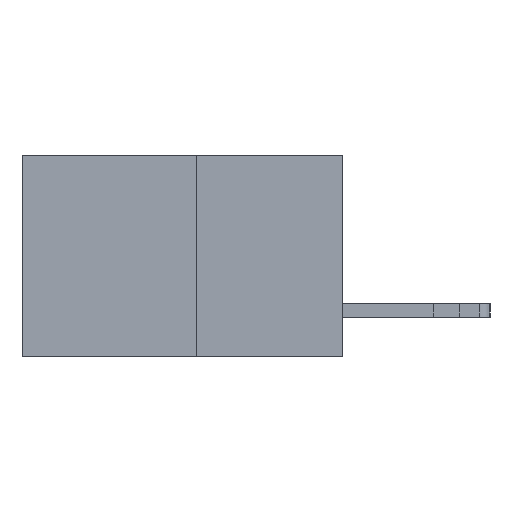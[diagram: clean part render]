
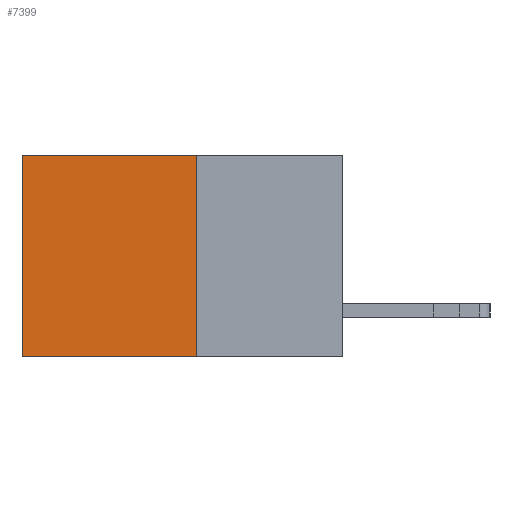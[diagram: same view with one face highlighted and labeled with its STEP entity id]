
A CAD part, left-side view. The second image highlights one B-rep face of the part: STEP entity #7399.
In plain terms, the highlighted planar face has unit normal (-1, 0, 0).
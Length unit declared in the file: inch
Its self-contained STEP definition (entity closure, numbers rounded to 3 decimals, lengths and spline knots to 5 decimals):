
#207 = VECTOR ( 'NONE', #7858, 39.37008 ) ;
#418 = CARTESIAN_POINT ( 'NONE',  ( 0.277, 0.59, 0. ) ) ;
#1033 = VECTOR ( 'NONE', #6911, 39.37008 ) ;
#1538 = CARTESIAN_POINT ( 'NONE',  ( 0.277, 0.59, -0.37 ) ) ;
#1669 = VECTOR ( 'NONE', #11132, 39.37008 ) ;
#1723 = DIRECTION ( 'NONE',  ( 0., 0., -1. ) ) ;
#2860 = VERTEX_POINT ( 'NONE', #6935 ) ;
#4498 = VECTOR ( 'NONE', #1723, 39.37008 ) ;
#4567 = LINE ( 'NONE', #6218, #207 ) ;
#6032 = AXIS2_PLACEMENT_3D ( 'NONE', #19266, #19016, #18831 ) ;
#6218 = CARTESIAN_POINT ( 'NONE',  ( 0.277, 0.59, -0.37 ) ) ;
#6911 = DIRECTION ( 'NONE',  ( 0., 1., 0. ) ) ;
#6935 = CARTESIAN_POINT ( 'NONE',  ( 0.277, 0.27, -0.37 ) ) ;
#7399 = ADVANCED_FACE ( 'NONE', ( #11169 ), #20513, .F. ) ;
#7858 = DIRECTION ( 'NONE',  ( 0., 0., -1. ) ) ;
#8882 = LINE ( 'NONE', #11604, #4498 ) ;
#9417 = LINE ( 'NONE', #9487, #1669 ) ;
#9487 = CARTESIAN_POINT ( 'NONE',  ( 0.277, 0.27, -0.37 ) ) ;
#9797 = VERTEX_POINT ( 'NONE', #16506 ) ;
#9915 = EDGE_CURVE ( 'NONE', #9797, #10580, #18491, .T. ) ;
#10374 = VERTEX_POINT ( 'NONE', #1538 ) ;
#10580 = VERTEX_POINT ( 'NONE', #418 ) ;
#11132 = DIRECTION ( 'NONE',  ( 0., 1., 0. ) ) ;
#11169 = FACE_OUTER_BOUND ( 'NONE', #18157, .T. ) ;
#11604 = CARTESIAN_POINT ( 'NONE',  ( 0.277, 0.27, -0.37 ) ) ;
#12090 = EDGE_CURVE ( 'NONE', #10580, #10374, #4567, .T. ) ;
#13515 = CARTESIAN_POINT ( 'NONE',  ( 0.277, 0.27, 0. ) ) ;
#13606 = ORIENTED_EDGE ( 'NONE', *, *, #14935, .F. ) ;
#14935 = EDGE_CURVE ( 'NONE', #9797, #2860, #8882, .T. ) ;
#16506 = CARTESIAN_POINT ( 'NONE',  ( 0.277, 0.27, 0. ) ) ;
#17117 = ORIENTED_EDGE ( 'NONE', *, *, #18791, .F. ) ;
#17186 = ORIENTED_EDGE ( 'NONE', *, *, #12090, .T. ) ;
#18157 = EDGE_LOOP ( 'NONE', ( #17186, #17117, #13606, #19272 ) ) ;
#18491 = LINE ( 'NONE', #13515, #1033 ) ;
#18791 = EDGE_CURVE ( 'NONE', #2860, #10374, #9417, .T. ) ;
#18831 = DIRECTION ( 'NONE',  ( 0., 0., -1. ) ) ;
#19016 = DIRECTION ( 'NONE',  ( 1., 0., 0. ) ) ;
#19266 = CARTESIAN_POINT ( 'NONE',  ( 0.277, 0.27, -0.37 ) ) ;
#19272 = ORIENTED_EDGE ( 'NONE', *, *, #9915, .T. ) ;
#20513 = PLANE ( 'NONE',  #6032 ) ;
